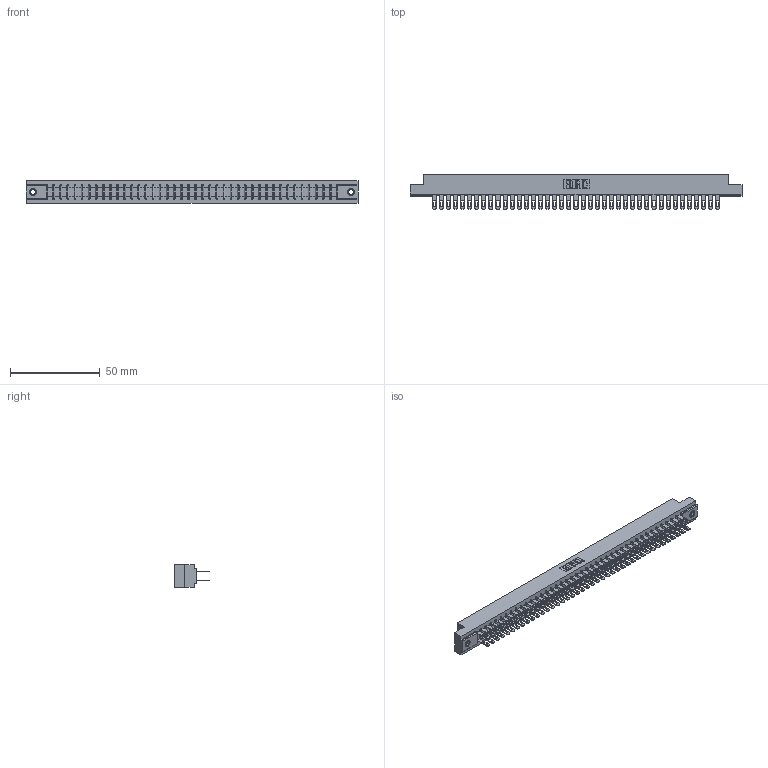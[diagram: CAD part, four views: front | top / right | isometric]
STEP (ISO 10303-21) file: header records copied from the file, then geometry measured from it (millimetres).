
FILE_DESCRIPTION (( 'STEP AP203' ), '1' );
FILE_NAME ('807-082-500-207.STEP', '2021-07-20T17:17:40', ( '' ), ( '' ), 'SwSTEP 2.0', 'SolidWorks 2020', '' );
FILE_SCHEMA (( 'CONFIG_CONTROL_DESIGN' ));
Length unit declared in the file: inch
Products named in the file (4): 307-290-001_500; 807-082-500-207; 345-250-001_345-250-005-103; 807 Part_.156 Dia Mounting Holes
Assembly tree (85 placements, depth 2):
  807-082-500-207
    807 Part_.156 Dia Mounting Holes
    307-290-001_500  x82
    345-250-001_345-250-005-103  x2
Bounding box: 185.47 x 19.18 x 12.7 mm (x, y, z)
Volume: 19937 mm3; surface area: 25712.1 mm2
Topology: 85 solids, 85 shells, 3992 faces, 11119 edges, 7182 vertices
Faces by surface type: plane 2562, cylinder 1330, sphere 84, cone 12, torus 4
Entity records: 37743 total; most frequent: CARTESIAN_POINT 6156, ORIENTED_EDGE 6094, DIRECTION 6041, EDGE_CURVE 3047, LINE 2335, VECTOR 2335, VERTEX_POINT 1968, AXIS2_PLACEMENT_3D 1853
